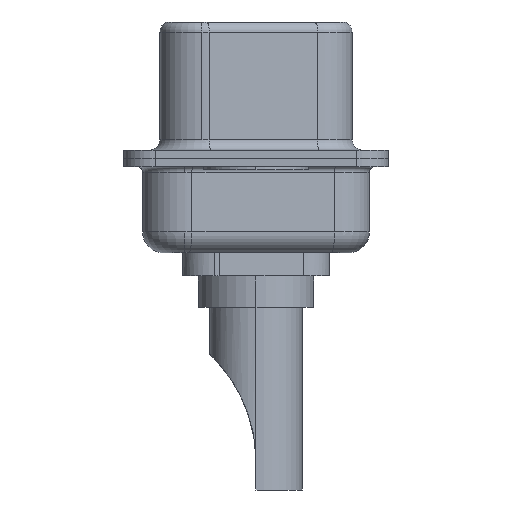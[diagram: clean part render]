
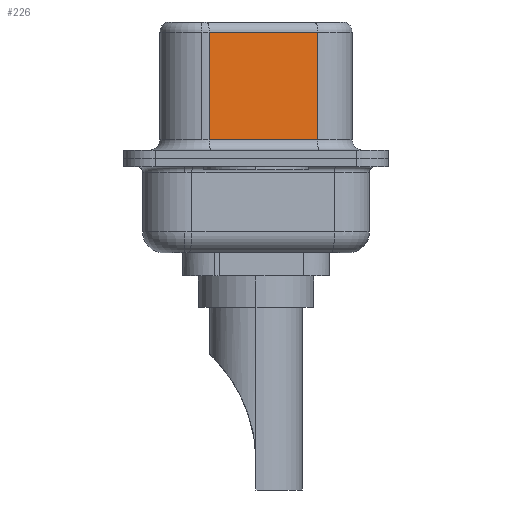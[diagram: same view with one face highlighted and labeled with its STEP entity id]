
A CAD part, left-side view. The second image highlights one B-rep face of the part: STEP entity #226.
In plain terms, the highlighted planar face has unit normal (-0.985, -0.174, 0).
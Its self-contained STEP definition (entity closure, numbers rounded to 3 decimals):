
#38 = EDGE_CURVE ( 'NONE', #3055, #10491, #7280, .T. ) ;
#226 = ADVANCED_FACE ( 'NONE', ( #5142 ), #9098, .F. ) ;
#397 = DIRECTION ( 'NONE',  ( 0.985, 0.174, 0. ) ) ;
#782 = ORIENTED_EDGE ( 'NONE', *, *, #914, .T. ) ;
#914 = EDGE_CURVE ( 'NONE', #4401, #5628, #12005, .T. ) ;
#1277 = EDGE_CURVE ( 'NONE', #5628, #3055, #9930, .T. ) ;
#2036 = ORIENTED_EDGE ( 'NONE', *, *, #1277, .T. ) ;
#2780 = CARTESIAN_POINT ( 'NONE',  ( 4.585, -2.927, 0.9 ) ) ;
#3055 = VERTEX_POINT ( 'NONE', #11408 ) ;
#3465 = CARTESIAN_POINT ( 'NONE',  ( 4.585, -2.927, 6.52 ) ) ;
#3578 = ORIENTED_EDGE ( 'NONE', *, *, #38, .T. ) ;
#4401 = VERTEX_POINT ( 'NONE', #8649 ) ;
#4561 = CARTESIAN_POINT ( 'NONE',  ( 4.585, -2.927, 6.52 ) ) ;
#4734 = CARTESIAN_POINT ( 'NONE',  ( 4.585, -2.927, 0.9 ) ) ;
#5142 = FACE_OUTER_BOUND ( 'NONE', #10168, .T. ) ;
#5367 = DIRECTION ( 'NONE',  ( 0., 0., -1. ) ) ;
#5561 = CARTESIAN_POINT ( 'NONE',  ( 4.585, -2.927, 6.02 ) ) ;
#5628 = VERTEX_POINT ( 'NONE', #8757 ) ;
#5728 = CARTESIAN_POINT ( 'NONE',  ( 3.675, 2.233, 6.52 ) ) ;
#6801 = VECTOR ( 'NONE', #5367, 1000. ) ;
#7110 = LINE ( 'NONE', #3465, #6801 ) ;
#7280 = LINE ( 'NONE', #2780, #11859 ) ;
#7970 = DIRECTION ( 'NONE',  ( -0.174, 0.985, 0. ) ) ;
#8324 = EDGE_CURVE ( 'NONE', #4401, #10491, #7110, .T. ) ;
#8649 = CARTESIAN_POINT ( 'NONE',  ( 4.585, -2.927, 6.02 ) ) ;
#8757 = CARTESIAN_POINT ( 'NONE',  ( 3.675, 2.233, 6.02 ) ) ;
#8781 = DIRECTION ( 'NONE',  ( -0.174, 0.985, 0. ) ) ;
#9098 = PLANE ( 'NONE',  #9927 ) ;
#9346 = VECTOR ( 'NONE', #8781, 1000. ) ;
#9606 = ORIENTED_EDGE ( 'NONE', *, *, #8324, .F. ) ;
#9927 = AXIS2_PLACEMENT_3D ( 'NONE', #4561, #397, #7970 ) ;
#9930 = LINE ( 'NONE', #5728, #12309 ) ;
#10017 = DIRECTION ( 'NONE',  ( 0., 0., -1. ) ) ;
#10168 = EDGE_LOOP ( 'NONE', ( #9606, #782, #2036, #3578 ) ) ;
#10491 = VERTEX_POINT ( 'NONE', #4734 ) ;
#10935 = DIRECTION ( 'NONE',  ( 0.174, -0.985, 0. ) ) ;
#11408 = CARTESIAN_POINT ( 'NONE',  ( 3.675, 2.233, 0.9 ) ) ;
#11859 = VECTOR ( 'NONE', #10935, 1000. ) ;
#12005 = LINE ( 'NONE', #5561, #9346 ) ;
#12309 = VECTOR ( 'NONE', #10017, 1000. ) ;
